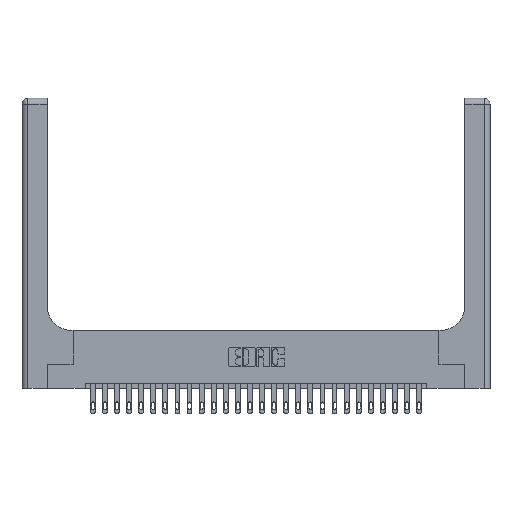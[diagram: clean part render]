
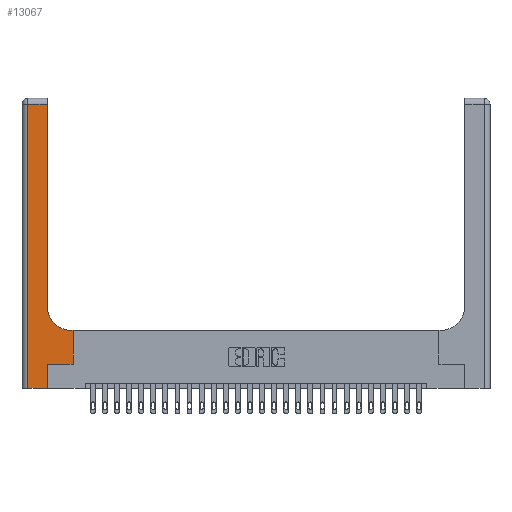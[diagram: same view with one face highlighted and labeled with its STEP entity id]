
A CAD part, top view. The second image highlights one B-rep face of the part: STEP entity #13067.
In plain terms, the highlighted planar face has unit normal (0, 0, 1).
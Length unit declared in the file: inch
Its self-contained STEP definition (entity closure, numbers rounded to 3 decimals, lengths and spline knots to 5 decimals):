
#39 = DIRECTION ( 'NONE',  ( 1., 0., 0. ) ) ;
#267 = FACE_OUTER_BOUND ( 'NONE', #13848, .T. ) ;
#424 = ORIENTED_EDGE ( 'NONE', *, *, #12881, .T. ) ;
#451 = VECTOR ( 'NONE', #3383, 39.37008 ) ;
#567 = DIRECTION ( 'NONE',  ( -1., 0., 0. ) ) ;
#743 = VERTEX_POINT ( 'NONE', #1653 ) ;
#885 = VERTEX_POINT ( 'NONE', #2305 ) ;
#1271 = DIRECTION ( 'NONE',  ( 1., 0., 0. ) ) ;
#1484 = CARTESIAN_POINT ( 'NONE',  ( 0.528, 0.25, 0.37 ) ) ;
#1653 = CARTESIAN_POINT ( 'NONE',  ( 0.51, 0.6, 0.37 ) ) ;
#1862 = CARTESIAN_POINT ( 'NONE',  ( 0.265, 0.25, 0.37 ) ) ;
#2159 = VERTEX_POINT ( 'NONE', #12214 ) ;
#2305 = CARTESIAN_POINT ( 'NONE',  ( 0.06, 2.94, 0.37 ) ) ;
#2899 = CARTESIAN_POINT ( 'NONE',  ( 0.265, 0.25, 0.37 ) ) ;
#3383 = DIRECTION ( 'NONE',  ( -1., 0., 0. ) ) ;
#3645 = DIRECTION ( 'NONE',  ( 0., 1., 0. ) ) ;
#3731 = EDGE_CURVE ( 'NONE', #885, #19375, #15716, .T. ) ;
#4020 = VECTOR ( 'NONE', #1271, 39.37008 ) ;
#4063 = CARTESIAN_POINT ( 'NONE',  ( 0.51, 0.85, 0.37 ) ) ;
#5162 = ORIENTED_EDGE ( 'NONE', *, *, #3731, .T. ) ;
#5261 = DIRECTION ( 'NONE',  ( 0., 1., 0. ) ) ;
#5454 = CARTESIAN_POINT ( 'NONE',  ( 0., 2.94, 0.37 ) ) ;
#5778 = CARTESIAN_POINT ( 'NONE',  ( 0.06, 0., 0.37 ) ) ;
#6289 = VECTOR ( 'NONE', #567, 39.37008 ) ;
#6968 = VECTOR ( 'NONE', #3645, 39.37008 ) ;
#7278 = VERTEX_POINT ( 'NONE', #23793 ) ;
#7427 = CARTESIAN_POINT ( 'NONE',  ( 0.528, 0.25, 0.37 ) ) ;
#7728 = LINE ( 'NONE', #9944, #8984 ) ;
#7839 = LINE ( 'NONE', #1862, #22499 ) ;
#8194 = PLANE ( 'NONE',  #16419 ) ;
#8354 = DIRECTION ( 'NONE',  ( 1., 0., 0. ) ) ;
#8359 = VERTEX_POINT ( 'NONE', #20581 ) ;
#8523 = ORIENTED_EDGE ( 'NONE', *, *, #18818, .T. ) ;
#8984 = VECTOR ( 'NONE', #9561, 39.37008 ) ;
#9232 = ORIENTED_EDGE ( 'NONE', *, *, #9389, .T. ) ;
#9301 = CARTESIAN_POINT ( 'NONE',  ( 0.265, 0., 0.37 ) ) ;
#9389 = EDGE_CURVE ( 'NONE', #15767, #19480, #17388, .T. ) ;
#9475 = ORIENTED_EDGE ( 'NONE', *, *, #9632, .T. ) ;
#9561 = DIRECTION ( 'NONE',  ( 0., 1., 0. ) ) ;
#9632 = EDGE_CURVE ( 'NONE', #8359, #743, #12673, .T. ) ;
#9944 = CARTESIAN_POINT ( 'NONE',  ( 0.26, 3., 0.37 ) ) ;
#11003 = EDGE_CURVE ( 'NONE', #19480, #25403, #7839, .T. ) ;
#11057 = LINE ( 'NONE', #5454, #451 ) ;
#11072 = LINE ( 'NONE', #7427, #6968 ) ;
#11265 = VECTOR ( 'NONE', #5261, 39.37008 ) ;
#11871 = CARTESIAN_POINT ( 'NONE',  ( 0.265, 0., 0.37 ) ) ;
#11939 = CARTESIAN_POINT ( 'NONE',  ( 0.06, 3., 0.37 ) ) ;
#12153 = ORIENTED_EDGE ( 'NONE', *, *, #18677, .T. ) ;
#12214 = CARTESIAN_POINT ( 'NONE',  ( 0.26, 0.85, 0.37 ) ) ;
#12673 = LINE ( 'NONE', #22159, #6289 ) ;
#12881 = EDGE_CURVE ( 'NONE', #25403, #8359, #11072, .T. ) ;
#13067 = ADVANCED_FACE ( 'NONE', ( #267 ), #8194, .F. ) ;
#13128 = LINE ( 'NONE', #17312, #4020 ) ;
#13848 = EDGE_LOOP ( 'NONE', ( #16260, #15291, #5162, #8523, #9232, #17387, #424, #9475, #12153 ) ) ;
#14200 = DIRECTION ( 'NONE',  ( -1., 0., 0. ) ) ;
#15291 = ORIENTED_EDGE ( 'NONE', *, *, #23394, .T. ) ;
#15716 = LINE ( 'NONE', #11939, #17682 ) ;
#15767 = VERTEX_POINT ( 'NONE', #11871 ) ;
#16150 = DIRECTION ( 'NONE',  ( 0., 0., -1. ) ) ;
#16260 = ORIENTED_EDGE ( 'NONE', *, *, #18232, .T. ) ;
#16419 = AXIS2_PLACEMENT_3D ( 'NONE', #24075, #16150, #14200 ) ;
#16506 = AXIS2_PLACEMENT_3D ( 'NONE', #4063, #18138, #8354 ) ;
#17312 = CARTESIAN_POINT ( 'NONE',  ( 0., 0., 0.37 ) ) ;
#17387 = ORIENTED_EDGE ( 'NONE', *, *, #11003, .T. ) ;
#17388 = LINE ( 'NONE', #9301, #11265 ) ;
#17682 = VECTOR ( 'NONE', #23504, 39.37008 ) ;
#18138 = DIRECTION ( 'NONE',  ( 0., 0., -1. ) ) ;
#18232 = EDGE_CURVE ( 'NONE', #2159, #7278, #7728, .T. ) ;
#18677 = EDGE_CURVE ( 'NONE', #743, #2159, #22289, .T. ) ;
#18818 = EDGE_CURVE ( 'NONE', #19375, #15767, #13128, .T. ) ;
#19375 = VERTEX_POINT ( 'NONE', #5778 ) ;
#19480 = VERTEX_POINT ( 'NONE', #2899 ) ;
#20581 = CARTESIAN_POINT ( 'NONE',  ( 0.528, 0.6, 0.37 ) ) ;
#22159 = CARTESIAN_POINT ( 'NONE',  ( 0.26, 0.6, 0.37 ) ) ;
#22289 = CIRCLE ( 'NONE', #16506, 0.25 ) ;
#22499 = VECTOR ( 'NONE', #39, 39.37008 ) ;
#23394 = EDGE_CURVE ( 'NONE', #7278, #885, #11057, .T. ) ;
#23504 = DIRECTION ( 'NONE',  ( 0., -1., 0. ) ) ;
#23793 = CARTESIAN_POINT ( 'NONE',  ( 0.26, 2.94, 0.37 ) ) ;
#24075 = CARTESIAN_POINT ( 'NONE',  ( 0., 3., 0.37 ) ) ;
#25403 = VERTEX_POINT ( 'NONE', #1484 ) ;
